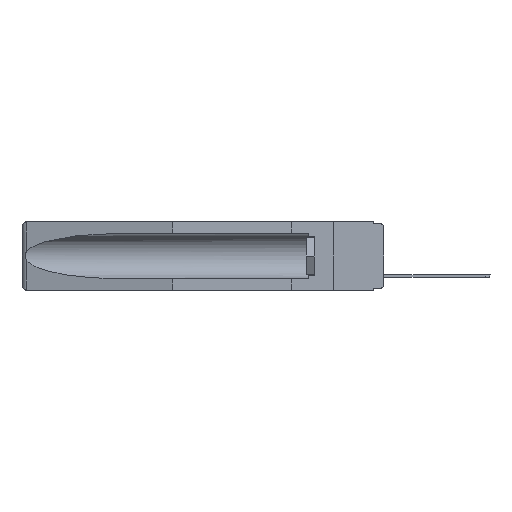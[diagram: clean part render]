
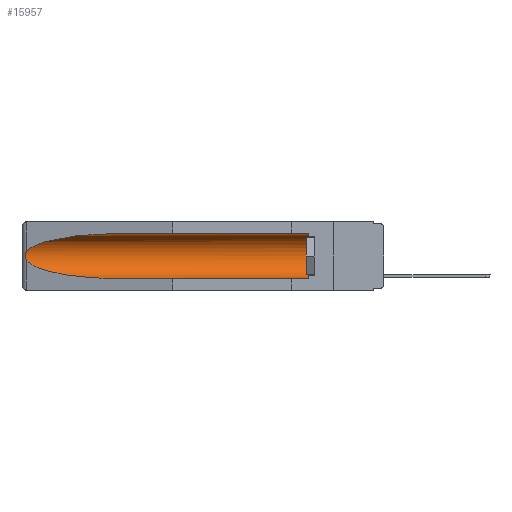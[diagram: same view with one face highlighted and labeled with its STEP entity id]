
A CAD part, left-side view. The second image highlights one B-rep face of the part: STEP entity #15957.
In plain terms, the highlighted cylindrical face has radius 2.857 mm (diameter 5.715 mm), a partial arc.
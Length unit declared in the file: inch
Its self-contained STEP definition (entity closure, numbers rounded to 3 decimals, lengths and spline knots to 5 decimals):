
#604 = CARTESIAN_POINT ( 'NONE',  ( 0.26597, 1.5296, -0.19026 ) ) ;
#663 = VERTEX_POINT ( 'NONE', #15926 ) ;
#771 = EDGE_CURVE ( 'NONE', #8878, #663, #16986, .T. ) ;
#989 = ORIENTED_EDGE ( 'NONE', *, *, #2216, .F. ) ;
#2058 = CARTESIAN_POINT ( 'NONE',  ( 0.26537, 1.52718, -0.19328 ) ) ;
#2216 = EDGE_CURVE ( 'NONE', #8878, #8730, #8051, .T. ) ;
#2342 = CARTESIAN_POINT ( 'NONE',  ( 0.21114, 1.30732, -0.059 ) ) ;
#2763 = DIRECTION ( 'NONE',  ( 0., 0., 1. ) ) ;
#2946 = VERTEX_POINT ( 'NONE', #12002 ) ;
#3253 = B_SPLINE_CURVE_WITH_KNOTS ( 'NONE', 3,
 ( #9801, #17415, #8260, #3771, #17324, #14674, #8155, #16006, #604, #2058 ),
 .UNSPECIFIED., .F., .F.,
 ( 4, 2, 2, 2, 4 ),
 ( 0., 0.00029, 0.00058, 0.00087, 0.00117 ),
 .UNSPECIFIED. ) ;
#3568 = VECTOR ( 'NONE', #17169, 39.37008 ) ;
#3641 = AXIS2_PLACEMENT_3D ( 'NONE', #15284, #15592, #2763 ) ;
#3771 = CARTESIAN_POINT ( 'NONE',  ( 0.2673, 1.5327, -0.16383 ) ) ;
#4115 = EDGE_CURVE ( 'NONE', #663, #6795, #6160, .T. ) ;
#4157 = CARTESIAN_POINT ( 'NONE',  ( 0.26537, 1.52718, -0.14972 ) ) ;
#4580 = CARTESIAN_POINT ( 'NONE',  ( 0.155, -0.30754, -0.1715 ) ) ;
#4748 = CARTESIAN_POINT ( 'NONE',  ( 0.26537, 1.52718, -0.19328 ) ) ;
#5753 = ORIENTED_EDGE ( 'NONE', *, *, #771, .T. ) ;
#6048 = CARTESIAN_POINT ( 'NONE',  ( 0.155, 1.07973, -0.284 ) ) ;
#6054 = CARTESIAN_POINT ( 'NONE',  ( 0.155, -0.30754, -0.059 ) ) ;
#6160 = LINE ( 'NONE', #6054, #3568 ) ;
#6360 = CARTESIAN_POINT ( 'NONE',  ( 0.25451, 1.48313, -0.24835 ) ) ;
#6684 = EDGE_CURVE ( 'NONE', #2946, #17454, #3253, .T. ) ;
#6795 = VERTEX_POINT ( 'NONE', #11629 ) ;
#6803 = CARTESIAN_POINT ( 'NONE',  ( 0.26537, 1.52718, -0.19328 ) ) ;
#7001 = CARTESIAN_POINT ( 'NONE',  ( 0.25451, 1.48313, -0.09465 ) ) ;
#7694 = CARTESIAN_POINT ( 'NONE',  ( 0.21114, 1.30732, -0.284 ) ) ;
#7695 = ORIENTED_EDGE ( 'NONE', *, *, #16290, .T. ) ;
#8051 = LINE ( 'NONE', #17025, #15460 ) ;
#8155 = CARTESIAN_POINT ( 'NONE',  ( 0.2673, 1.53269, -0.17917 ) ) ;
#8260 = CARTESIAN_POINT ( 'NONE',  ( 0.26654, 1.53092, -0.15636 ) ) ;
#8730 = VERTEX_POINT ( 'NONE', #6048 ) ;
#8878 = VERTEX_POINT ( 'NONE', #11497 ) ;
#9343 =( BOUNDED_CURVE ( )  B_SPLINE_CURVE ( 3, ( #4748, #6360, #7694, #16857 ),
 .UNSPECIFIED., .F., .T. ) 
 B_SPLINE_CURVE_WITH_KNOTS ( ( 4, 4 ),
 ( 0.1948, 1.5708 ),
 .UNSPECIFIED. ) 
 CURVE ( )  GEOMETRIC_REPRESENTATION_ITEM ( )  RATIONAL_B_SPLINE_CURVE ( ( 1., 0.848, 0.848, 1. ) ) 
 REPRESENTATION_ITEM ( '' )  );
#9772 = AXIS2_PLACEMENT_3D ( 'NONE', #4580, #10926, #18218 ) ;
#9801 = CARTESIAN_POINT ( 'NONE',  ( 0.26537, 1.52718, -0.14972 ) ) ;
#10821 = FACE_OUTER_BOUND ( 'NONE', #19399, .T. ) ;
#10926 = DIRECTION ( 'NONE',  ( 0., 1., 0. ) ) ;
#11401 =( BOUNDED_CURVE ( )  B_SPLINE_CURVE ( 3, ( #11722, #2342, #7001, #4157 ),
 .UNSPECIFIED., .F., .T. ) 
 B_SPLINE_CURVE_WITH_KNOTS ( ( 4, 4 ),
 ( 4.71239, 6.08839 ),
 .UNSPECIFIED. ) 
 CURVE ( )  GEOMETRIC_REPRESENTATION_ITEM ( )  RATIONAL_B_SPLINE_CURVE ( ( 1., 0.848, 0.848, 1. ) ) 
 REPRESENTATION_ITEM ( '' )  );
#11478 = ORIENTED_EDGE ( 'NONE', *, *, #6684, .T. ) ;
#11497 = CARTESIAN_POINT ( 'NONE',  ( 0.155, 0.126, -0.284 ) ) ;
#11629 = CARTESIAN_POINT ( 'NONE',  ( 0.155, 1.07973, -0.059 ) ) ;
#11722 = CARTESIAN_POINT ( 'NONE',  ( 0.155, 1.07973, -0.059 ) ) ;
#12002 = CARTESIAN_POINT ( 'NONE',  ( 0.26537, 1.52718, -0.14972 ) ) ;
#13136 = EDGE_CURVE ( 'NONE', #17454, #8730, #9343, .T. ) ;
#14674 = CARTESIAN_POINT ( 'NONE',  ( 0.2675, 1.53308, -0.17534 ) ) ;
#14791 = ORIENTED_EDGE ( 'NONE', *, *, #13136, .T. ) ;
#15284 = CARTESIAN_POINT ( 'NONE',  ( 0.155, 0.126, -0.1715 ) ) ;
#15460 = VECTOR ( 'NONE', #15899, 39.37008 ) ;
#15480 = CYLINDRICAL_SURFACE ( 'NONE', #9772, 0.1125 ) ;
#15592 = DIRECTION ( 'NONE',  ( 0., -1., 0. ) ) ;
#15899 = DIRECTION ( 'NONE',  ( 0., 1., 0. ) ) ;
#15926 = CARTESIAN_POINT ( 'NONE',  ( 0.155, 0.126, -0.059 ) ) ;
#15957 = ADVANCED_FACE ( 'NONE', ( #10821 ), #15480, .F. ) ;
#16006 = CARTESIAN_POINT ( 'NONE',  ( 0.26655, 1.53094, -0.18657 ) ) ;
#16290 = EDGE_CURVE ( 'NONE', #6795, #2946, #11401, .T. ) ;
#16847 = ORIENTED_EDGE ( 'NONE', *, *, #4115, .T. ) ;
#16857 = CARTESIAN_POINT ( 'NONE',  ( 0.155, 1.07973, -0.284 ) ) ;
#16986 = CIRCLE ( 'NONE', #3641, 0.1125 ) ;
#17025 = CARTESIAN_POINT ( 'NONE',  ( 0.155, -0.30754, -0.284 ) ) ;
#17169 = DIRECTION ( 'NONE',  ( 0., 1., 0. ) ) ;
#17324 = CARTESIAN_POINT ( 'NONE',  ( 0.2675, 1.53308, -0.16763 ) ) ;
#17415 = CARTESIAN_POINT ( 'NONE',  ( 0.26597, 1.52961, -0.15275 ) ) ;
#17454 = VERTEX_POINT ( 'NONE', #6803 ) ;
#18218 = DIRECTION ( 'NONE',  ( 0., 0., 1. ) ) ;
#19399 = EDGE_LOOP ( 'NONE', ( #7695, #11478, #14791, #989, #5753, #16847 ) ) ;
